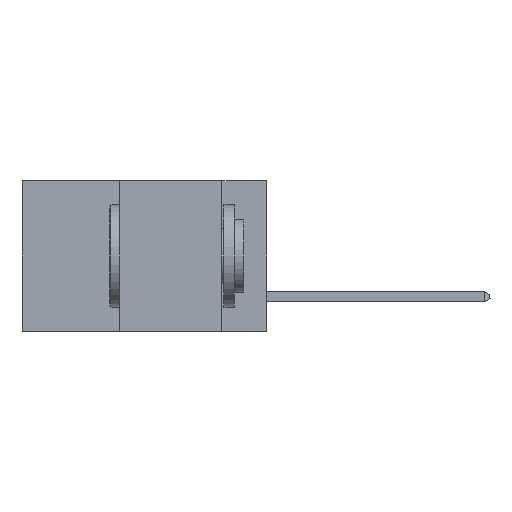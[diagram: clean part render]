
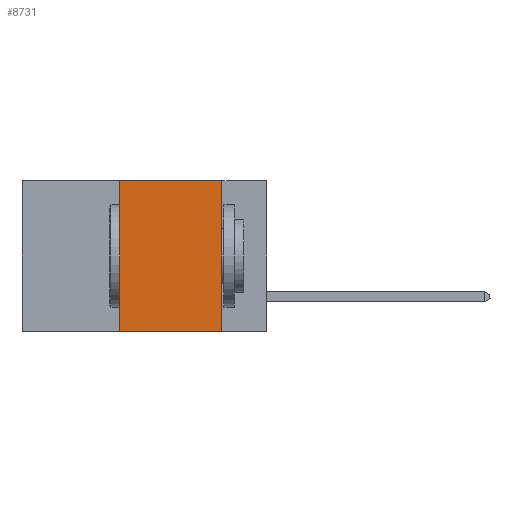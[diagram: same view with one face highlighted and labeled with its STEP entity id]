
A CAD part, left-side view. The second image highlights one B-rep face of the part: STEP entity #8731.
In plain terms, the highlighted planar face has unit normal (-1, 0, 0).
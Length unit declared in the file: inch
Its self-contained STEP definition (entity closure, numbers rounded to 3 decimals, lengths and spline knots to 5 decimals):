
#592 = FACE_OUTER_BOUND ( 'NONE', #21555, .T. ) ;
#751 = DIRECTION ( 'NONE',  ( 0., 0., 1. ) ) ;
#1044 = VECTOR ( 'NONE', #18652, 39.37008 ) ;
#3411 = LINE ( 'NONE', #24513, #13273 ) ;
#3845 = ORIENTED_EDGE ( 'NONE', *, *, #6133, .F. ) ;
#6133 = EDGE_CURVE ( 'NONE', #17597, #10445, #21726, .T. ) ;
#6822 = CARTESIAN_POINT ( 'NONE',  ( 0., 0.6, 0. ) ) ;
#7022 = EDGE_CURVE ( 'NONE', #19630, #9135, #24072, .T. ) ;
#7767 = CARTESIAN_POINT ( 'NONE',  ( 0., 0.11, 0. ) ) ;
#8731 = ADVANCED_FACE ( 'NONE', ( #592 ), #18961, .F. ) ;
#9135 = VERTEX_POINT ( 'NONE', #23718 ) ;
#9543 = VECTOR ( 'NONE', #19674, 39.37008 ) ;
#10445 = VERTEX_POINT ( 'NONE', #23087 ) ;
#10927 = ORIENTED_EDGE ( 'NONE', *, *, #11432, .F. ) ;
#11432 = EDGE_CURVE ( 'NONE', #10445, #9135, #23295, .T. ) ;
#11986 = CARTESIAN_POINT ( 'NONE',  ( 0., 0.36, 0. ) ) ;
#13273 = VECTOR ( 'NONE', #751, 39.37008 ) ;
#17542 = ORIENTED_EDGE ( 'NONE', *, *, #23128, .F. ) ;
#17597 = VERTEX_POINT ( 'NONE', #11986 ) ;
#18652 = DIRECTION ( 'NONE',  ( 0., -1., 0. ) ) ;
#18961 = PLANE ( 'NONE',  #21997 ) ;
#19053 = DIRECTION ( 'NONE',  ( 0., 0., -1. ) ) ;
#19571 = VECTOR ( 'NONE', #24735, 39.37008 ) ;
#19630 = VERTEX_POINT ( 'NONE', #27713 ) ;
#19674 = DIRECTION ( 'NONE',  ( 0., -1., 0. ) ) ;
#21184 = ORIENTED_EDGE ( 'NONE', *, *, #7022, .T. ) ;
#21555 = EDGE_LOOP ( 'NONE', ( #10927, #3845, #17542, #21184 ) ) ;
#21726 = LINE ( 'NONE', #6822, #9543 ) ;
#21997 = AXIS2_PLACEMENT_3D ( 'NONE', #25747, #23434, #19053 ) ;
#22923 = CARTESIAN_POINT ( 'NONE',  ( 0., 0.6, -0.37 ) ) ;
#23087 = CARTESIAN_POINT ( 'NONE',  ( 0., 0.11, 0. ) ) ;
#23128 = EDGE_CURVE ( 'NONE', #19630, #17597, #3411, .T. ) ;
#23295 = LINE ( 'NONE', #7767, #19571 ) ;
#23434 = DIRECTION ( 'NONE',  ( 1., 0., 0. ) ) ;
#23718 = CARTESIAN_POINT ( 'NONE',  ( 0., 0.11, -0.37 ) ) ;
#24072 = LINE ( 'NONE', #22923, #1044 ) ;
#24513 = CARTESIAN_POINT ( 'NONE',  ( 0., 0.36, 0. ) ) ;
#24735 = DIRECTION ( 'NONE',  ( 0., 0., -1. ) ) ;
#25747 = CARTESIAN_POINT ( 'NONE',  ( 0., 0.6, 0. ) ) ;
#27713 = CARTESIAN_POINT ( 'NONE',  ( 0., 0.36, -0.37 ) ) ;
